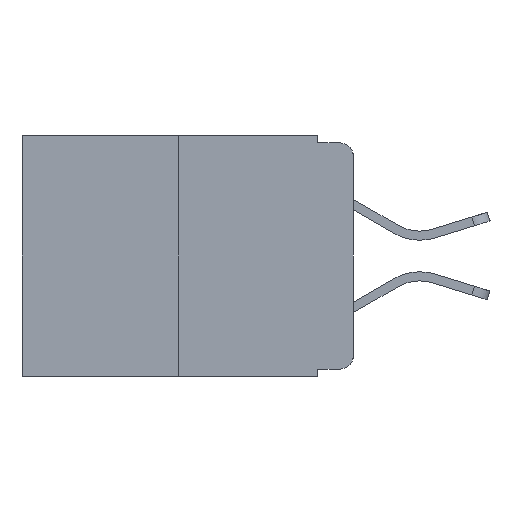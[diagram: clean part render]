
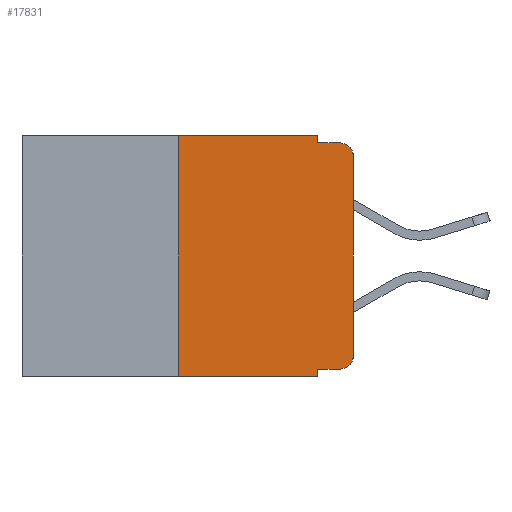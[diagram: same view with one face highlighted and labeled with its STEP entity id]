
A CAD part, left-side view. The second image highlights one B-rep face of the part: STEP entity #17831.
In plain terms, the highlighted planar face has unit normal (-1, 0, 0).
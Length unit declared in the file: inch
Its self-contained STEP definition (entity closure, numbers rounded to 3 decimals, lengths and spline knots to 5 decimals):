
#70 = ORIENTED_EDGE ( 'NONE', *, *, #9290, .F. ) ;
#123 = DIRECTION ( 'NONE',  ( 0., -1., 0. ) ) ;
#210 = ORIENTED_EDGE ( 'NONE', *, *, #12556, .T. ) ;
#808 = LINE ( 'NONE', #9965, #13807 ) ;
#1028 = DIRECTION ( 'NONE',  ( -1., 0., 0. ) ) ;
#1142 = VERTEX_POINT ( 'NONE', #16396 ) ;
#1216 = ORIENTED_EDGE ( 'NONE', *, *, #20618, .F. ) ;
#1659 = ORIENTED_EDGE ( 'NONE', *, *, #13139, .F. ) ;
#1755 = LINE ( 'NONE', #15121, #17925 ) ;
#1912 = EDGE_CURVE ( 'NONE', #1142, #12986, #2608, .T. ) ;
#1917 = VERTEX_POINT ( 'NONE', #8781 ) ;
#2038 = ORIENTED_EDGE ( 'NONE', *, *, #1912, .F. ) ;
#2123 = VECTOR ( 'NONE', #18301, 39.37008 ) ;
#2272 = CIRCLE ( 'NONE', #12691, 0.02 ) ;
#2378 = DIRECTION ( 'NONE',  ( 0., 0., -1. ) ) ;
#2608 = LINE ( 'NONE', #3137, #10740 ) ;
#3062 = CARTESIAN_POINT ( 'NONE',  ( 0., 0.051, -0.01 ) ) ;
#3074 = VERTEX_POINT ( 'NONE', #10412 ) ;
#3137 = CARTESIAN_POINT ( 'NONE',  ( 0., 0.25, 0. ) ) ;
#3341 = VECTOR ( 'NONE', #6761, 39.37008 ) ;
#3372 = ORIENTED_EDGE ( 'NONE', *, *, #4009, .T. ) ;
#4009 = EDGE_CURVE ( 'NONE', #5823, #16393, #2272, .T. ) ;
#4193 = ORIENTED_EDGE ( 'NONE', *, *, #18410, .T. ) ;
#4533 = AXIS2_PLACEMENT_3D ( 'NONE', #10812, #1028, #12450 ) ;
#4866 = VECTOR ( 'NONE', #17574, 39.37008 ) ;
#5285 = CARTESIAN_POINT ( 'NONE',  ( 0., 0.473, 0. ) ) ;
#5472 = DIRECTION ( 'NONE',  ( 0., -1., 0. ) ) ;
#5823 = VERTEX_POINT ( 'NONE', #7569 ) ;
#6028 = LINE ( 'NONE', #12110, #9813 ) ;
#6375 = CARTESIAN_POINT ( 'NONE',  ( 0., 0.02, -0.333 ) ) ;
#6761 = DIRECTION ( 'NONE',  ( 0., 0., 1. ) ) ;
#6791 = CARTESIAN_POINT ( 'NONE',  ( 0., 0.02, -0.03 ) ) ;
#7569 = CARTESIAN_POINT ( 'NONE',  ( 0., 0., -0.03 ) ) ;
#7939 = CIRCLE ( 'NONE', #4533, 0.02 ) ;
#7941 = DIRECTION ( 'NONE',  ( 0., 0., -1. ) ) ;
#8137 = AXIS2_PLACEMENT_3D ( 'NONE', #5285, #19715, #10147 ) ;
#8470 = ORIENTED_EDGE ( 'NONE', *, *, #18527, .T. ) ;
#8781 = CARTESIAN_POINT ( 'NONE',  ( 0., 0.051, 0. ) ) ;
#9105 = VERTEX_POINT ( 'NONE', #11626 ) ;
#9167 = LINE ( 'NONE', #3062, #4866 ) ;
#9290 = EDGE_CURVE ( 'NONE', #1917, #10806, #6028, .T. ) ;
#9813 = VECTOR ( 'NONE', #2378, 39.37008 ) ;
#9965 = CARTESIAN_POINT ( 'NONE',  ( 0., 0.473, 0. ) ) ;
#10147 = DIRECTION ( 'NONE',  ( 0., 0., -1. ) ) ;
#10219 = VERTEX_POINT ( 'NONE', #14283 ) ;
#10412 = CARTESIAN_POINT ( 'NONE',  ( 0., 0., -0.313 ) ) ;
#10417 = EDGE_CURVE ( 'NONE', #12986, #1917, #808, .T. ) ;
#10570 = EDGE_CURVE ( 'NONE', #1142, #9105, #15048, .T. ) ;
#10740 = VECTOR ( 'NONE', #19460, 39.37008 ) ;
#10806 = VERTEX_POINT ( 'NONE', #17323 ) ;
#10812 = CARTESIAN_POINT ( 'NONE',  ( 0., 0.02, -0.313 ) ) ;
#11419 = LINE ( 'NONE', #15959, #19885 ) ;
#11626 = CARTESIAN_POINT ( 'NONE',  ( 0., 0.051, -0.343 ) ) ;
#11999 = CARTESIAN_POINT ( 'NONE',  ( 0., 0.25, 0. ) ) ;
#12110 = CARTESIAN_POINT ( 'NONE',  ( 0., 0.051, 0. ) ) ;
#12333 = ORIENTED_EDGE ( 'NONE', *, *, #10570, .T. ) ;
#12450 = DIRECTION ( 'NONE',  ( 0., 0., -1. ) ) ;
#12556 = EDGE_CURVE ( 'NONE', #19686, #3074, #7939, .T. ) ;
#12691 = AXIS2_PLACEMENT_3D ( 'NONE', #6791, #16756, #17271 ) ;
#12986 = VERTEX_POINT ( 'NONE', #11999 ) ;
#13139 = EDGE_CURVE ( 'NONE', #10806, #16393, #9167, .T. ) ;
#13522 = EDGE_LOOP ( 'NONE', ( #4193, #3372, #1659, #70, #19633, #2038, #12333, #1216, #8470, #210 ) ) ;
#13807 = VECTOR ( 'NONE', #123, 39.37008 ) ;
#14283 = CARTESIAN_POINT ( 'NONE',  ( 0., 0.051, -0.333 ) ) ;
#15048 = LINE ( 'NONE', #16712, #2123 ) ;
#15121 = CARTESIAN_POINT ( 'NONE',  ( 0., 0.051, -0.333 ) ) ;
#15959 = CARTESIAN_POINT ( 'NONE',  ( 0., 0.051, 0. ) ) ;
#16206 = LINE ( 'NONE', #19555, #3341 ) ;
#16393 = VERTEX_POINT ( 'NONE', #18719 ) ;
#16396 = CARTESIAN_POINT ( 'NONE',  ( 0., 0.25, -0.343 ) ) ;
#16539 = PLANE ( 'NONE',  #8137 ) ;
#16712 = CARTESIAN_POINT ( 'NONE',  ( 0., 0.473, -0.343 ) ) ;
#16756 = DIRECTION ( 'NONE',  ( -1., 0., 0. ) ) ;
#17271 = DIRECTION ( 'NONE',  ( 0., 0., -1. ) ) ;
#17323 = CARTESIAN_POINT ( 'NONE',  ( 0., 0.051, -0.01 ) ) ;
#17574 = DIRECTION ( 'NONE',  ( 0., -1., 0. ) ) ;
#17831 = ADVANCED_FACE ( 'NONE', ( #19197 ), #16539, .F. ) ;
#17925 = VECTOR ( 'NONE', #5472, 39.37008 ) ;
#18301 = DIRECTION ( 'NONE',  ( 0., -1., 0. ) ) ;
#18410 = EDGE_CURVE ( 'NONE', #3074, #5823, #16206, .T. ) ;
#18527 = EDGE_CURVE ( 'NONE', #10219, #19686, #1755, .T. ) ;
#18719 = CARTESIAN_POINT ( 'NONE',  ( 0., 0.02, -0.01 ) ) ;
#19197 = FACE_OUTER_BOUND ( 'NONE', #13522, .T. ) ;
#19460 = DIRECTION ( 'NONE',  ( 0., 0., 1. ) ) ;
#19555 = CARTESIAN_POINT ( 'NONE',  ( 0., 0., 0. ) ) ;
#19633 = ORIENTED_EDGE ( 'NONE', *, *, #10417, .F. ) ;
#19686 = VERTEX_POINT ( 'NONE', #6375 ) ;
#19715 = DIRECTION ( 'NONE',  ( 1., 0., 0. ) ) ;
#19885 = VECTOR ( 'NONE', #7941, 39.37008 ) ;
#20618 = EDGE_CURVE ( 'NONE', #10219, #9105, #11419, .T. ) ;
